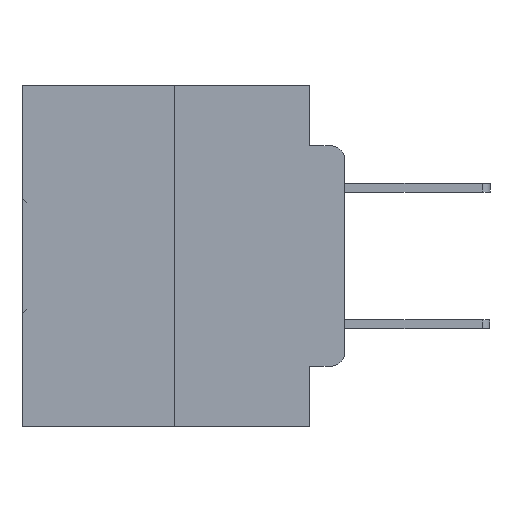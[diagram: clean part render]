
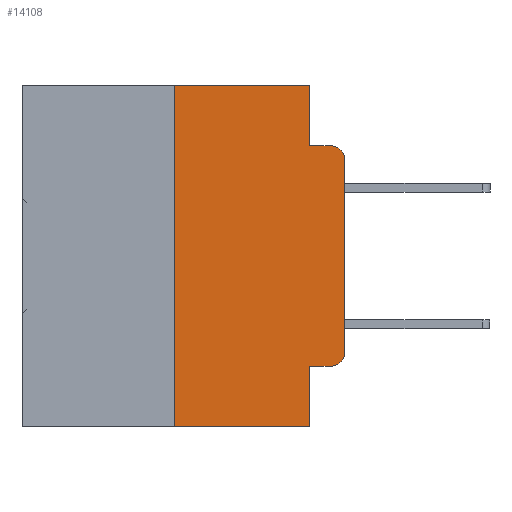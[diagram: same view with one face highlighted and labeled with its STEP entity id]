
A CAD part, left-side view. The second image highlights one B-rep face of the part: STEP entity #14108.
In plain terms, the highlighted planar face has unit normal (-1, 0, 0).
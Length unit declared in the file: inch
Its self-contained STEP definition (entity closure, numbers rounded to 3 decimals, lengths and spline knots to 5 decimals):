
#77 = CARTESIAN_POINT ( 'NONE',  ( 0., 0.051, 0. ) ) ;
#1042 = CARTESIAN_POINT ( 'NONE',  ( 0., 0.051, -0.4115 ) ) ;
#1051 = CARTESIAN_POINT ( 'NONE',  ( 0., 0.473, 0. ) ) ;
#1339 = DIRECTION ( 'NONE',  ( -1., 0., 0. ) ) ;
#2278 = VECTOR ( 'NONE', #28786, 39.37008 ) ;
#2366 = CARTESIAN_POINT ( 'NONE',  ( 0., 0.02, -0.3915 ) ) ;
#2639 = ORIENTED_EDGE ( 'NONE', *, *, #21221, .T. ) ;
#2661 = EDGE_CURVE ( 'NONE', #8464, #27394, #14462, .T. ) ;
#3785 = VERTEX_POINT ( 'NONE', #20119 ) ;
#4387 = CARTESIAN_POINT ( 'NONE',  ( 0., 0.25, 0. ) ) ;
#4416 = CARTESIAN_POINT ( 'NONE',  ( 0., 0.051, -0.4115 ) ) ;
#5073 = DIRECTION ( 'NONE',  ( 0., 0., -1. ) ) ;
#5115 = VECTOR ( 'NONE', #29428, 39.37008 ) ;
#5209 = EDGE_CURVE ( 'NONE', #29740, #23538, #33155, .T. ) ;
#5494 = DIRECTION ( 'NONE',  ( 0., 0., -1. ) ) ;
#5598 = LINE ( 'NONE', #1051, #25920 ) ;
#6495 = DIRECTION ( 'NONE',  ( 0., -1., 0. ) ) ;
#7338 = CARTESIAN_POINT ( 'NONE',  ( 0., 0.25, -0.5 ) ) ;
#7605 = ORIENTED_EDGE ( 'NONE', *, *, #17222, .F. ) ;
#7713 = EDGE_CURVE ( 'NONE', #21556, #8339, #8495, .T. ) ;
#7982 = ORIENTED_EDGE ( 'NONE', *, *, #14597, .T. ) ;
#8051 = CARTESIAN_POINT ( 'NONE',  ( 0., 0., -0.1085 ) ) ;
#8339 = VERTEX_POINT ( 'NONE', #18607 ) ;
#8464 = VERTEX_POINT ( 'NONE', #24480 ) ;
#8495 = LINE ( 'NONE', #16061, #14683 ) ;
#9128 = EDGE_LOOP ( 'NONE', ( #33801, #7982, #7605, #22705, #30790, #15942, #13636, #11376, #22431, #2639 ) ) ;
#9431 = LINE ( 'NONE', #26183, #2278 ) ;
#9439 = LINE ( 'NONE', #33714, #27996 ) ;
#10766 = VECTOR ( 'NONE', #18799, 39.37008 ) ;
#11376 = ORIENTED_EDGE ( 'NONE', *, *, #7713, .F. ) ;
#12462 = EDGE_CURVE ( 'NONE', #29740, #8339, #9431, .T. ) ;
#12482 = DIRECTION ( 'NONE',  ( 0., 0., -1. ) ) ;
#12769 = LINE ( 'NONE', #4416, #26796 ) ;
#12990 = CIRCLE ( 'NONE', #26211, 0.02 ) ;
#13636 = ORIENTED_EDGE ( 'NONE', *, *, #12462, .T. ) ;
#13671 = CARTESIAN_POINT ( 'NONE',  ( 0., 0.25, 0. ) ) ;
#14108 = ADVANCED_FACE ( 'NONE', ( #26584 ), #25533, .F. ) ;
#14462 = LINE ( 'NONE', #18362, #27659 ) ;
#14597 = EDGE_CURVE ( 'NONE', #27394, #27954, #17086, .T. ) ;
#14683 = VECTOR ( 'NONE', #5494, 39.37008 ) ;
#15251 = AXIS2_PLACEMENT_3D ( 'NONE', #17337, #1339, #20053 ) ;
#15497 = EDGE_CURVE ( 'NONE', #16807, #3785, #30936, .T. ) ;
#15942 = ORIENTED_EDGE ( 'NONE', *, *, #5209, .F. ) ;
#16061 = CARTESIAN_POINT ( 'NONE',  ( 0., 0.051, 0. ) ) ;
#16335 = CARTESIAN_POINT ( 'NONE',  ( 0., 0.051, 0. ) ) ;
#16807 = VERTEX_POINT ( 'NONE', #16335 ) ;
#17086 = CIRCLE ( 'NONE', #15251, 0.02 ) ;
#17222 = EDGE_CURVE ( 'NONE', #3785, #27954, #9439, .T. ) ;
#17337 = CARTESIAN_POINT ( 'NONE',  ( 0., 0.02, -0.1085 ) ) ;
#18362 = CARTESIAN_POINT ( 'NONE',  ( 0., 0., 0. ) ) ;
#18607 = CARTESIAN_POINT ( 'NONE',  ( 0., 0.051, -0.5 ) ) ;
#18633 = DIRECTION ( 'NONE',  ( 0., 0., 1. ) ) ;
#18799 = DIRECTION ( 'NONE',  ( 0., 0., -1. ) ) ;
#19598 = EDGE_CURVE ( 'NONE', #23538, #16807, #5598, .T. ) ;
#20053 = DIRECTION ( 'NONE',  ( 0., 0., -1. ) ) ;
#20119 = CARTESIAN_POINT ( 'NONE',  ( 0., 0.051, -0.0885 ) ) ;
#21042 = DIRECTION ( 'NONE',  ( -1., 0., 0. ) ) ;
#21221 = EDGE_CURVE ( 'NONE', #22884, #8464, #12990, .T. ) ;
#21556 = VERTEX_POINT ( 'NONE', #1042 ) ;
#22431 = ORIENTED_EDGE ( 'NONE', *, *, #24843, .T. ) ;
#22705 = ORIENTED_EDGE ( 'NONE', *, *, #15497, .F. ) ;
#22884 = VERTEX_POINT ( 'NONE', #33473 ) ;
#23050 = CARTESIAN_POINT ( 'NONE',  ( 0., 0.473, 0. ) ) ;
#23538 = VERTEX_POINT ( 'NONE', #4387 ) ;
#24294 = DIRECTION ( 'NONE',  ( 0., -1., 0. ) ) ;
#24480 = CARTESIAN_POINT ( 'NONE',  ( 0., 0., -0.3915 ) ) ;
#24843 = EDGE_CURVE ( 'NONE', #21556, #22884, #12769, .T. ) ;
#25533 = PLANE ( 'NONE',  #28904 ) ;
#25920 = VECTOR ( 'NONE', #6495, 39.37008 ) ;
#26183 = CARTESIAN_POINT ( 'NONE',  ( 0., 0.473, -0.5 ) ) ;
#26211 = AXIS2_PLACEMENT_3D ( 'NONE', #2366, #21042, #5073 ) ;
#26249 = CARTESIAN_POINT ( 'NONE',  ( 0., 0.02, -0.0885 ) ) ;
#26584 = FACE_OUTER_BOUND ( 'NONE', #9128, .T. ) ;
#26796 = VECTOR ( 'NONE', #24294, 39.37008 ) ;
#27394 = VERTEX_POINT ( 'NONE', #8051 ) ;
#27659 = VECTOR ( 'NONE', #18633, 39.37008 ) ;
#27954 = VERTEX_POINT ( 'NONE', #26249 ) ;
#27996 = VECTOR ( 'NONE', #28599, 39.37008 ) ;
#28270 = DIRECTION ( 'NONE',  ( 1., 0., 0. ) ) ;
#28599 = DIRECTION ( 'NONE',  ( 0., -1., 0. ) ) ;
#28786 = DIRECTION ( 'NONE',  ( 0., -1., 0. ) ) ;
#28904 = AXIS2_PLACEMENT_3D ( 'NONE', #23050, #28270, #12482 ) ;
#29428 = DIRECTION ( 'NONE',  ( 0., 0., 1. ) ) ;
#29740 = VERTEX_POINT ( 'NONE', #7338 ) ;
#30790 = ORIENTED_EDGE ( 'NONE', *, *, #19598, .F. ) ;
#30936 = LINE ( 'NONE', #77, #10766 ) ;
#33155 = LINE ( 'NONE', #13671, #5115 ) ;
#33473 = CARTESIAN_POINT ( 'NONE',  ( 0., 0.02, -0.4115 ) ) ;
#33714 = CARTESIAN_POINT ( 'NONE',  ( 0., 0.051, -0.0885 ) ) ;
#33801 = ORIENTED_EDGE ( 'NONE', *, *, #2661, .T. ) ;
